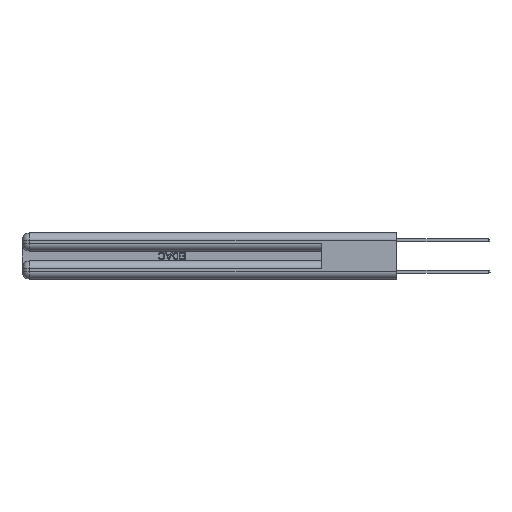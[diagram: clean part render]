
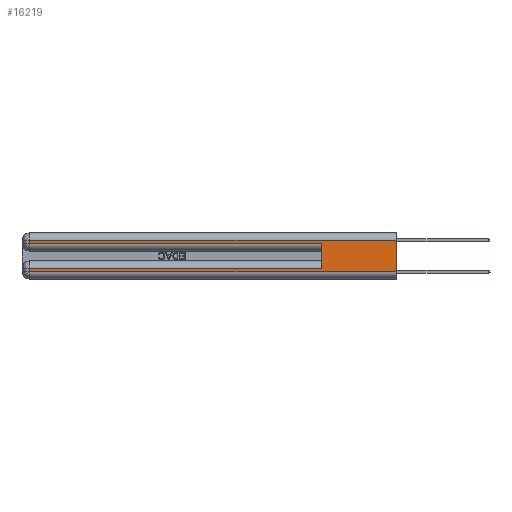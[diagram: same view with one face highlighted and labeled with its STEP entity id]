
A CAD part, left-side view. The second image highlights one B-rep face of the part: STEP entity #16219.
In plain terms, the highlighted planar face has unit normal (-1, 0, 0).
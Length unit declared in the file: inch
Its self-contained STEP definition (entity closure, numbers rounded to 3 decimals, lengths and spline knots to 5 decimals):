
#195 = ORIENTED_EDGE ( 'NONE', *, *, #3078, .T. ) ;
#216 = LINE ( 'NONE', #11693, #30175 ) ;
#1090 = CARTESIAN_POINT ( 'NONE',  ( 0., 0., 0.37 ) ) ;
#1603 = CARTESIAN_POINT ( 'NONE',  ( 0., 2.94, 0.37 ) ) ;
#1867 = VECTOR ( 'NONE', #25048, 39.37008 ) ;
#2163 = CARTESIAN_POINT ( 'NONE',  ( 0., 2.94, 0.085 ) ) ;
#3018 = ORIENTED_EDGE ( 'NONE', *, *, #16156, .T. ) ;
#3078 = EDGE_CURVE ( 'NONE', #26610, #21673, #216, .T. ) ;
#4580 = ORIENTED_EDGE ( 'NONE', *, *, #25632, .T. ) ;
#4581 = CARTESIAN_POINT ( 'NONE',  ( 0., 0.6, 0.285 ) ) ;
#5378 = CARTESIAN_POINT ( 'NONE',  ( 0., 0., 0.085 ) ) ;
#5899 = FACE_OUTER_BOUND ( 'NONE', #11200, .T. ) ;
#6300 = DIRECTION ( 'NONE',  ( 0., -1., 0. ) ) ;
#6812 = CARTESIAN_POINT ( 'NONE',  ( 0., 2.94, 0.37 ) ) ;
#7476 = EDGE_CURVE ( 'NONE', #29783, #21619, #16521, .T. ) ;
#7556 = CARTESIAN_POINT ( 'NONE',  ( 0., 0., 0.06 ) ) ;
#7574 = VERTEX_POINT ( 'NONE', #12383 ) ;
#9044 = CARTESIAN_POINT ( 'NONE',  ( 0., 0., 0.31 ) ) ;
#9888 = ORIENTED_EDGE ( 'NONE', *, *, #31566, .T. ) ;
#9969 = CARTESIAN_POINT ( 'NONE',  ( 0., 0., 0.37 ) ) ;
#9990 = CARTESIAN_POINT ( 'NONE',  ( 0., 0., 0.285 ) ) ;
#10083 = DIRECTION ( 'NONE',  ( 0., 0., -1. ) ) ;
#10567 = AXIS2_PLACEMENT_3D ( 'NONE', #9969, #27634, #10083 ) ;
#11200 = EDGE_LOOP ( 'NONE', ( #30521, #28535, #3018, #12269, #31019, #4580, #9888, #195 ) ) ;
#11693 = CARTESIAN_POINT ( 'NONE',  ( 0., 0., 0.06 ) ) ;
#11735 = CARTESIAN_POINT ( 'NONE',  ( 0., 2.94, 0.06 ) ) ;
#11759 = VERTEX_POINT ( 'NONE', #29718 ) ;
#12090 = DIRECTION ( 'NONE',  ( 0., -1., 0. ) ) ;
#12266 = VECTOR ( 'NONE', #32251, 39.37008 ) ;
#12269 = ORIENTED_EDGE ( 'NONE', *, *, #24477, .T. ) ;
#12383 = CARTESIAN_POINT ( 'NONE',  ( 0., 2.94, 0.285 ) ) ;
#12517 = VECTOR ( 'NONE', #17255, 39.37008 ) ;
#14444 = DIRECTION ( 'NONE',  ( 0., 1., 0. ) ) ;
#15748 = LINE ( 'NONE', #9990, #22469 ) ;
#16156 = EDGE_CURVE ( 'NONE', #24010, #7574, #29218, .T. ) ;
#16219 = ADVANCED_FACE ( 'NONE', ( #5899 ), #25113, .F. ) ;
#16499 = CARTESIAN_POINT ( 'NONE',  ( 0., 2.94, 0.31 ) ) ;
#16521 = LINE ( 'NONE', #22279, #12517 ) ;
#16877 = VECTOR ( 'NONE', #28637, 39.37008 ) ;
#17255 = DIRECTION ( 'NONE',  ( 0., 0., 1. ) ) ;
#17394 = VECTOR ( 'NONE', #19281, 39.37008 ) ;
#19281 = DIRECTION ( 'NONE',  ( 0., 0., -1. ) ) ;
#19901 = EDGE_CURVE ( 'NONE', #11759, #21673, #29840, .T. ) ;
#21619 = VERTEX_POINT ( 'NONE', #4581 ) ;
#21673 = VERTEX_POINT ( 'NONE', #7556 ) ;
#22279 = CARTESIAN_POINT ( 'NONE',  ( 0., 0.6, 0.145 ) ) ;
#22469 = VECTOR ( 'NONE', #12090, 39.37008 ) ;
#22850 = LINE ( 'NONE', #9044, #23654 ) ;
#23654 = VECTOR ( 'NONE', #14444, 39.37008 ) ;
#24010 = VERTEX_POINT ( 'NONE', #16499 ) ;
#24477 = EDGE_CURVE ( 'NONE', #7574, #21619, #15748, .T. ) ;
#25048 = DIRECTION ( 'NONE',  ( 0., 1., 0. ) ) ;
#25113 = PLANE ( 'NONE',  #10567 ) ;
#25632 = EDGE_CURVE ( 'NONE', #29783, #32572, #27134, .T. ) ;
#26610 = VERTEX_POINT ( 'NONE', #11735 ) ;
#26969 = EDGE_CURVE ( 'NONE', #11759, #24010, #22850, .T. ) ;
#27134 = LINE ( 'NONE', #5378, #1867 ) ;
#27634 = DIRECTION ( 'NONE',  ( 1., 0., 0. ) ) ;
#28535 = ORIENTED_EDGE ( 'NONE', *, *, #26969, .T. ) ;
#28637 = DIRECTION ( 'NONE',  ( 0., 0., -1. ) ) ;
#29218 = LINE ( 'NONE', #1603, #17394 ) ;
#29718 = CARTESIAN_POINT ( 'NONE',  ( 0., 0., 0.31 ) ) ;
#29783 = VERTEX_POINT ( 'NONE', #31690 ) ;
#29840 = LINE ( 'NONE', #1090, #16877 ) ;
#30175 = VECTOR ( 'NONE', #6300, 39.37008 ) ;
#30424 = LINE ( 'NONE', #6812, #12266 ) ;
#30521 = ORIENTED_EDGE ( 'NONE', *, *, #19901, .F. ) ;
#31019 = ORIENTED_EDGE ( 'NONE', *, *, #7476, .F. ) ;
#31566 = EDGE_CURVE ( 'NONE', #32572, #26610, #30424, .T. ) ;
#31690 = CARTESIAN_POINT ( 'NONE',  ( 0., 0.6, 0.085 ) ) ;
#32251 = DIRECTION ( 'NONE',  ( 0., 0., -1. ) ) ;
#32572 = VERTEX_POINT ( 'NONE', #2163 ) ;
